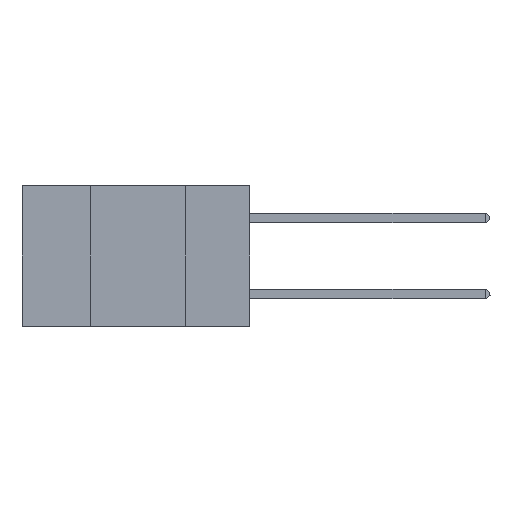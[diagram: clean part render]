
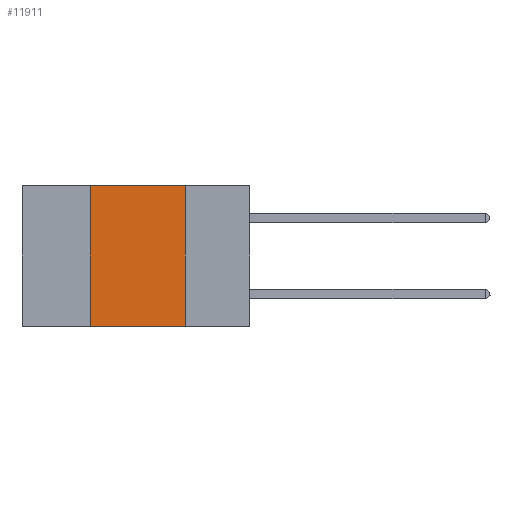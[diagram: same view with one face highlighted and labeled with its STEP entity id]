
A CAD part, left-side view. The second image highlights one B-rep face of the part: STEP entity #11911.
In plain terms, the highlighted planar face has unit normal (-1, 0, 0).
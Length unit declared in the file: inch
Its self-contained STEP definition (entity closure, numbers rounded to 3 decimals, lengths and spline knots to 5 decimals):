
#11 = ORIENTED_EDGE ( 'NONE', *, *, #7396, .F. ) ;
#199 = EDGE_CURVE ( 'NONE', #4305, #15131, #450, .T. ) ;
#450 = LINE ( 'NONE', #2553, #1180 ) ;
#772 = DIRECTION ( 'NONE',  ( 0., 0., -1. ) ) ;
#1105 = CARTESIAN_POINT ( 'NONE',  ( 0., 0.17, -0.37 ) ) ;
#1180 = VECTOR ( 'NONE', #15014, 39.37008 ) ;
#1434 = VERTEX_POINT ( 'NONE', #3914 ) ;
#1465 = EDGE_CURVE ( 'NONE', #4305, #1434, #1612, .T. ) ;
#1612 = LINE ( 'NONE', #11788, #8885 ) ;
#2553 = CARTESIAN_POINT ( 'NONE',  ( 0., 0.6, -0.37 ) ) ;
#3209 = VERTEX_POINT ( 'NONE', #3308 ) ;
#3308 = CARTESIAN_POINT ( 'NONE',  ( 0., 0.17, 0. ) ) ;
#3914 = CARTESIAN_POINT ( 'NONE',  ( 0., 0.42, 0. ) ) ;
#4305 = VERTEX_POINT ( 'NONE', #18728 ) ;
#4839 = CARTESIAN_POINT ( 'NONE',  ( 0., 0.6, 0. ) ) ;
#6865 = DIRECTION ( 'NONE',  ( 1., 0., 0. ) ) ;
#7026 = AXIS2_PLACEMENT_3D ( 'NONE', #14783, #6865, #772 ) ;
#7396 = EDGE_CURVE ( 'NONE', #3209, #15131, #17796, .T. ) ;
#7652 = ORIENTED_EDGE ( 'NONE', *, *, #1465, .F. ) ;
#8023 = VECTOR ( 'NONE', #10882, 39.37008 ) ;
#8366 = PLANE ( 'NONE',  #7026 ) ;
#8885 = VECTOR ( 'NONE', #16282, 39.37008 ) ;
#9502 = VECTOR ( 'NONE', #19703, 39.37008 ) ;
#10505 = EDGE_LOOP ( 'NONE', ( #11, #11413, #7652, #18467 ) ) ;
#10882 = DIRECTION ( 'NONE',  ( 0., -1., 0. ) ) ;
#11413 = ORIENTED_EDGE ( 'NONE', *, *, #18861, .F. ) ;
#11788 = CARTESIAN_POINT ( 'NONE',  ( 0., 0.42, 0. ) ) ;
#11911 = ADVANCED_FACE ( 'NONE', ( #16371 ), #8366, .F. ) ;
#14783 = CARTESIAN_POINT ( 'NONE',  ( 0., 0.6, 0. ) ) ;
#15014 = DIRECTION ( 'NONE',  ( 0., -1., 0. ) ) ;
#15131 = VERTEX_POINT ( 'NONE', #1105 ) ;
#15369 = LINE ( 'NONE', #4839, #8023 ) ;
#16282 = DIRECTION ( 'NONE',  ( 0., 0., 1. ) ) ;
#16371 = FACE_OUTER_BOUND ( 'NONE', #10505, .T. ) ;
#17796 = LINE ( 'NONE', #19291, #9502 ) ;
#18467 = ORIENTED_EDGE ( 'NONE', *, *, #199, .T. ) ;
#18728 = CARTESIAN_POINT ( 'NONE',  ( 0., 0.42, -0.37 ) ) ;
#18861 = EDGE_CURVE ( 'NONE', #1434, #3209, #15369, .T. ) ;
#19291 = CARTESIAN_POINT ( 'NONE',  ( 0., 0.17, 0. ) ) ;
#19703 = DIRECTION ( 'NONE',  ( 0., 0., -1. ) ) ;
